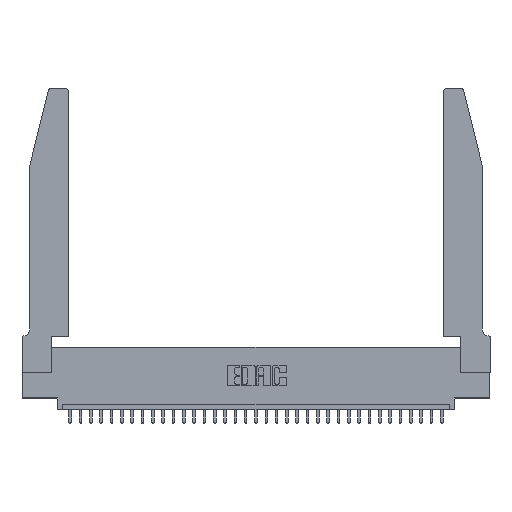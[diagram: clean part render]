
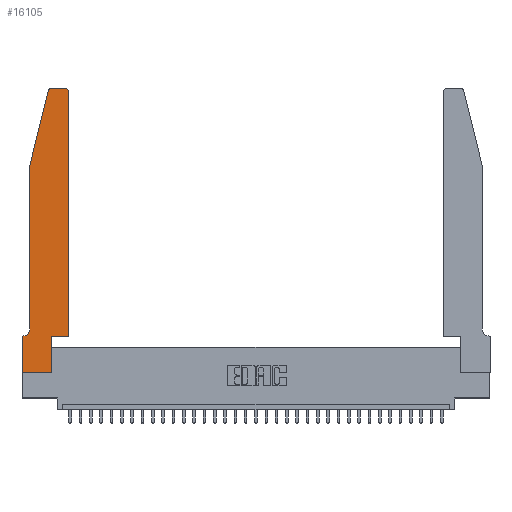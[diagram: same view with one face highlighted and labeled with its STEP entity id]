
A CAD part, top view. The second image highlights one B-rep face of the part: STEP entity #16105.
In plain terms, the highlighted planar face has unit normal (0, 0, 1).
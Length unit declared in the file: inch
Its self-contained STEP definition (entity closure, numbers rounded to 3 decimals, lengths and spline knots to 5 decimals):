
#575 = ORIENTED_EDGE ( 'NONE', *, *, #31806, .T. ) ;
#901 = ORIENTED_EDGE ( 'NONE', *, *, #9044, .T. ) ;
#1060 = ORIENTED_EDGE ( 'NONE', *, *, #27966, .T. ) ;
#1492 = EDGE_CURVE ( 'NONE', #5285, #10161, #25971, .T. ) ;
#1730 = LINE ( 'NONE', #19698, #26767 ) ;
#2031 = ORIENTED_EDGE ( 'NONE', *, *, #15135, .T. ) ;
#2192 = FACE_OUTER_BOUND ( 'NONE', #27727, .T. ) ;
#2969 = CARTESIAN_POINT ( 'NONE',  ( 0.0055, 0.42, 0.37 ) ) ;
#3313 = VECTOR ( 'NONE', #19736, 39.37008 ) ;
#3389 = ORIENTED_EDGE ( 'NONE', *, *, #1492, .T. ) ;
#3570 = CARTESIAN_POINT ( 'NONE',  ( 0., 0.35, 0.37 ) ) ;
#4668 = LINE ( 'NONE', #32474, #13121 ) ;
#4757 = CARTESIAN_POINT ( 'NONE',  ( 0.25487, 2.72718, 0.37 ) ) ;
#5122 = CARTESIAN_POINT ( 'NONE',  ( 0.4505, 0.35, 0.37 ) ) ;
#5285 = VERTEX_POINT ( 'NONE', #20987 ) ;
#5359 = CARTESIAN_POINT ( 'NONE',  ( 0.4505, 2.72, 0.37 ) ) ;
#5427 = LINE ( 'NONE', #26523, #11927 ) ;
#5811 = VECTOR ( 'NONE', #10904, 39.37008 ) ;
#7842 = VERTEX_POINT ( 'NONE', #10618 ) ;
#8341 = DIRECTION ( 'NONE',  ( -0.239, -0.971, 0. ) ) ;
#8423 = DIRECTION ( 'NONE',  ( -1., 0., 0. ) ) ;
#8536 = VERTEX_POINT ( 'NONE', #5359 ) ;
#8866 = DIRECTION ( 'NONE',  ( -1., 0., 0. ) ) ;
#9031 = CARTESIAN_POINT ( 'NONE',  ( 0.2865, 0.35, 0.37 ) ) ;
#9044 = EDGE_CURVE ( 'NONE', #30636, #24319, #1730, .T. ) ;
#9735 = AXIS2_PLACEMENT_3D ( 'NONE', #15733, #18344, #10519 ) ;
#9854 = CARTESIAN_POINT ( 'NONE',  ( 0., 0., 0.37 ) ) ;
#10113 = DIRECTION ( 'NONE',  ( 0., -1., 0. ) ) ;
#10161 = VERTEX_POINT ( 'NONE', #21486 ) ;
#10519 = DIRECTION ( 'NONE',  ( 1., 0., 0. ) ) ;
#10618 = CARTESIAN_POINT ( 'NONE',  ( 0.4205, 2.75, 0.37 ) ) ;
#10661 = DIRECTION ( 'NONE',  ( 0., 0., 1. ) ) ;
#10904 = DIRECTION ( 'NONE',  ( 0., 1., 0. ) ) ;
#11643 = CARTESIAN_POINT ( 'NONE',  ( 0.2605, 2.75, 0.37 ) ) ;
#11927 = VECTOR ( 'NONE', #8341, 39.37008 ) ;
#12371 = CARTESIAN_POINT ( 'NONE',  ( 0.2865, 0., 0.37 ) ) ;
#12457 = DIRECTION ( 'NONE',  ( 1., 0., 0. ) ) ;
#12928 = EDGE_CURVE ( 'NONE', #18393, #30636, #5427, .T. ) ;
#12995 = VERTEX_POINT ( 'NONE', #24180 ) ;
#13121 = VECTOR ( 'NONE', #10113, 39.37008 ) ;
#13145 = CIRCLE ( 'NONE', #9735, 0.03 ) ;
#13503 = DIRECTION ( 'NONE',  ( 1., 0., 0. ) ) ;
#13719 = CARTESIAN_POINT ( 'NONE',  ( 0.0755, 0.35, 0.37 ) ) ;
#13851 = DIRECTION ( 'NONE',  ( 0., 0., -1. ) ) ;
#14279 = VECTOR ( 'NONE', #8866, 39.37008 ) ;
#14528 = CARTESIAN_POINT ( 'NONE',  ( 0.2865, 0.35, 0.37 ) ) ;
#14657 = AXIS2_PLACEMENT_3D ( 'NONE', #28966, #10661, #13503 ) ;
#14749 = LINE ( 'NONE', #11643, #28451 ) ;
#14811 = DIRECTION ( 'NONE',  ( 0., -1., 0. ) ) ;
#15135 = EDGE_CURVE ( 'NONE', #12995, #31736, #22068, .T. ) ;
#15339 = EDGE_CURVE ( 'NONE', #10161, #12995, #4668, .T. ) ;
#15520 = VERTEX_POINT ( 'NONE', #23445 ) ;
#15646 = EDGE_CURVE ( 'NONE', #7842, #15520, #14749, .T. ) ;
#15668 = PLANE ( 'NONE',  #16118 ) ;
#15733 = CARTESIAN_POINT ( 'NONE',  ( 0.284, 2.72, 0.37 ) ) ;
#16105 = ADVANCED_FACE ( 'NONE', ( #2192 ), #15668, .T. ) ;
#16118 = AXIS2_PLACEMENT_3D ( 'NONE', #3570, #20316, #22674 ) ;
#17218 = EDGE_CURVE ( 'NONE', #31736, #18653, #27583, .T. ) ;
#18222 = VECTOR ( 'NONE', #33442, 39.37008 ) ;
#18344 = DIRECTION ( 'NONE',  ( 0., 0., 1. ) ) ;
#18393 = VERTEX_POINT ( 'NONE', #4757 ) ;
#18413 = ORIENTED_EDGE ( 'NONE', *, *, #15646, .T. ) ;
#18653 = VERTEX_POINT ( 'NONE', #9031 ) ;
#18844 = VECTOR ( 'NONE', #12457, 39.37008 ) ;
#19348 = ORIENTED_EDGE ( 'NONE', *, *, #21436, .T. ) ;
#19698 = CARTESIAN_POINT ( 'NONE',  ( 0.0755, 2., 0.37 ) ) ;
#19736 = DIRECTION ( 'NONE',  ( 0., 1., 0. ) ) ;
#19877 = LINE ( 'NONE', #5122, #18222 ) ;
#20316 = DIRECTION ( 'NONE',  ( 0., 0., 1. ) ) ;
#20436 = CARTESIAN_POINT ( 'NONE',  ( 0.0755, 0.42, 0.37 ) ) ;
#20451 = ORIENTED_EDGE ( 'NONE', *, *, #15339, .T. ) ;
#20949 = EDGE_CURVE ( 'NONE', #18653, #26997, #19877, .T. ) ;
#20987 = CARTESIAN_POINT ( 'NONE',  ( 0.0055, 0.35, 0.37 ) ) ;
#21436 = EDGE_CURVE ( 'NONE', #24319, #5285, #25081, .T. ) ;
#21486 = CARTESIAN_POINT ( 'NONE',  ( 0., 0.35, 0.37 ) ) ;
#22068 = LINE ( 'NONE', #9854, #18844 ) ;
#22674 = DIRECTION ( 'NONE',  ( 1., 0., 0. ) ) ;
#23445 = CARTESIAN_POINT ( 'NONE',  ( 0.284, 2.75, 0.37 ) ) ;
#24180 = CARTESIAN_POINT ( 'NONE',  ( 0., 0., 0.37 ) ) ;
#24255 = AXIS2_PLACEMENT_3D ( 'NONE', #2969, #13851, #8423 ) ;
#24319 = VERTEX_POINT ( 'NONE', #20436 ) ;
#25000 = ORIENTED_EDGE ( 'NONE', *, *, #20949, .T. ) ;
#25081 = CIRCLE ( 'NONE', #24255, 0.07 ) ;
#25971 = LINE ( 'NONE', #13719, #14279 ) ;
#26371 = CARTESIAN_POINT ( 'NONE',  ( 0.4505, 0.35, 0.37 ) ) ;
#26403 = LINE ( 'NONE', #26371, #5811 ) ;
#26523 = CARTESIAN_POINT ( 'NONE',  ( 0.0755, 2., 0.37 ) ) ;
#26767 = VECTOR ( 'NONE', #14811, 39.37008 ) ;
#26904 = DIRECTION ( 'NONE',  ( -1., 0., 0. ) ) ;
#26997 = VERTEX_POINT ( 'NONE', #27855 ) ;
#27026 = ORIENTED_EDGE ( 'NONE', *, *, #17218, .T. ) ;
#27583 = LINE ( 'NONE', #14528, #3313 ) ;
#27727 = EDGE_LOOP ( 'NONE', ( #18413, #575, #32454, #901, #19348, #3389, #20451, #2031, #27026, #25000, #33417, #1060 ) ) ;
#27855 = CARTESIAN_POINT ( 'NONE',  ( 0.4505, 0.35, 0.37 ) ) ;
#27965 = EDGE_CURVE ( 'NONE', #26997, #8536, #26403, .T. ) ;
#27966 = EDGE_CURVE ( 'NONE', #8536, #7842, #32470, .T. ) ;
#28451 = VECTOR ( 'NONE', #26904, 39.37008 ) ;
#28890 = CARTESIAN_POINT ( 'NONE',  ( 0.0755, 2., 0.37 ) ) ;
#28966 = CARTESIAN_POINT ( 'NONE',  ( 0.4205, 2.72, 0.37 ) ) ;
#30636 = VERTEX_POINT ( 'NONE', #28890 ) ;
#31736 = VERTEX_POINT ( 'NONE', #12371 ) ;
#31806 = EDGE_CURVE ( 'NONE', #15520, #18393, #13145, .T. ) ;
#32454 = ORIENTED_EDGE ( 'NONE', *, *, #12928, .T. ) ;
#32470 = CIRCLE ( 'NONE', #14657, 0.03 ) ;
#32474 = CARTESIAN_POINT ( 'NONE',  ( 0., 0., 0.37 ) ) ;
#33417 = ORIENTED_EDGE ( 'NONE', *, *, #27965, .T. ) ;
#33442 = DIRECTION ( 'NONE',  ( 1., 0., 0. ) ) ;
